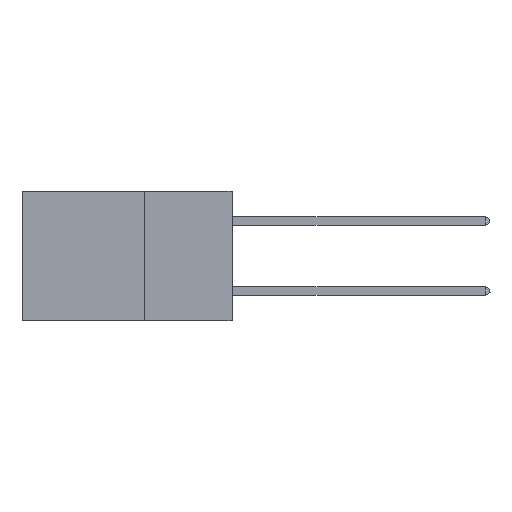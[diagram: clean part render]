
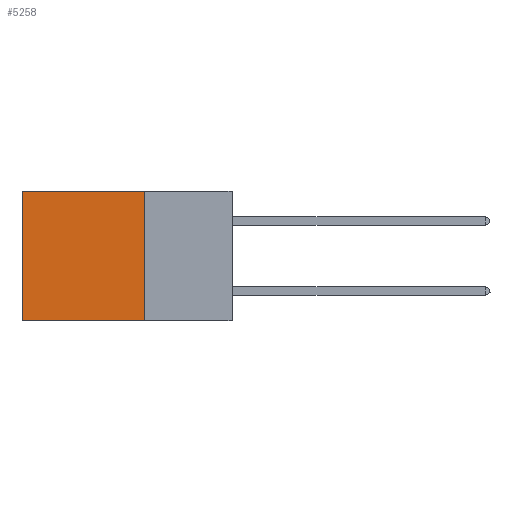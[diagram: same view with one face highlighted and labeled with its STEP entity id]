
A CAD part, left-side view. The second image highlights one B-rep face of the part: STEP entity #5258.
In plain terms, the highlighted planar face has unit normal (-1, 0, 0).
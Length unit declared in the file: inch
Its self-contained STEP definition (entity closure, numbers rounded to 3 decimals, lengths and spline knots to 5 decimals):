
#551 = DIRECTION ( 'NONE',  ( 0., 0., -1. ) ) ;
#660 = AXIS2_PLACEMENT_3D ( 'NONE', #10603, #2234, #551 ) ;
#726 = DIRECTION ( 'NONE',  ( 0., 1., 0. ) ) ;
#1855 = VERTEX_POINT ( 'NONE', #15602 ) ;
#2234 = DIRECTION ( 'NONE',  ( 1., 0., 0. ) ) ;
#5054 = DIRECTION ( 'NONE',  ( 0., 0., -1. ) ) ;
#5258 = ADVANCED_FACE ( 'NONE', ( #8882 ), #15969, .F. ) ;
#6253 = ORIENTED_EDGE ( 'NONE', *, *, #7922, .F. ) ;
#6453 = CARTESIAN_POINT ( 'NONE',  ( 0.2875, 0.6, 0. ) ) ;
#6533 = ORIENTED_EDGE ( 'NONE', *, *, #9577, .T. ) ;
#6687 = VECTOR ( 'NONE', #726, 39.37008 ) ;
#6911 = VECTOR ( 'NONE', #11706, 39.37008 ) ;
#7460 = VECTOR ( 'NONE', #5054, 39.37008 ) ;
#7740 = LINE ( 'NONE', #8604, #6687 ) ;
#7751 = CARTESIAN_POINT ( 'NONE',  ( 0.2875, 0.25, 0. ) ) ;
#7922 = EDGE_CURVE ( 'NONE', #1855, #11272, #16381, .T. ) ;
#8344 = EDGE_CURVE ( 'NONE', #1855, #16769, #16561, .T. ) ;
#8428 = EDGE_LOOP ( 'NONE', ( #6533, #9959, #6253, #11880 ) ) ;
#8604 = CARTESIAN_POINT ( 'NONE',  ( 0.2875, 0.25, -0.37 ) ) ;
#8670 = CARTESIAN_POINT ( 'NONE',  ( 0.2875, 0.25, 0. ) ) ;
#8882 = FACE_OUTER_BOUND ( 'NONE', #8428, .T. ) ;
#8987 = CARTESIAN_POINT ( 'NONE',  ( 0.2875, 0.6, -0.37 ) ) ;
#9577 = EDGE_CURVE ( 'NONE', #16769, #10984, #11910, .T. ) ;
#9959 = ORIENTED_EDGE ( 'NONE', *, *, #12121, .F. ) ;
#10603 = CARTESIAN_POINT ( 'NONE',  ( 0.2875, 0.25, 0. ) ) ;
#10689 = VECTOR ( 'NONE', #11618, 39.37008 ) ;
#10984 = VERTEX_POINT ( 'NONE', #8987 ) ;
#11272 = VERTEX_POINT ( 'NONE', #16621 ) ;
#11618 = DIRECTION ( 'NONE',  ( 0., 1., 0. ) ) ;
#11706 = DIRECTION ( 'NONE',  ( 0., 0., -1. ) ) ;
#11880 = ORIENTED_EDGE ( 'NONE', *, *, #8344, .T. ) ;
#11910 = LINE ( 'NONE', #6453, #7460 ) ;
#12121 = EDGE_CURVE ( 'NONE', #11272, #10984, #7740, .T. ) ;
#15602 = CARTESIAN_POINT ( 'NONE',  ( 0.2875, 0.25, 0. ) ) ;
#15658 = CARTESIAN_POINT ( 'NONE',  ( 0.2875, 0.6, 0. ) ) ;
#15969 = PLANE ( 'NONE',  #660 ) ;
#16381 = LINE ( 'NONE', #7751, #6911 ) ;
#16561 = LINE ( 'NONE', #8670, #10689 ) ;
#16621 = CARTESIAN_POINT ( 'NONE',  ( 0.2875, 0.25, -0.37 ) ) ;
#16769 = VERTEX_POINT ( 'NONE', #15658 ) ;
